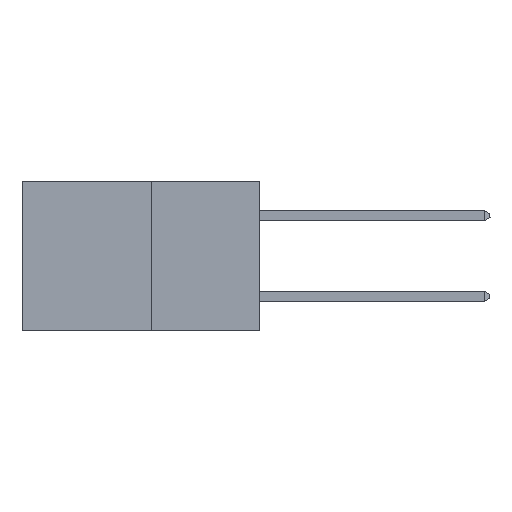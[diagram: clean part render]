
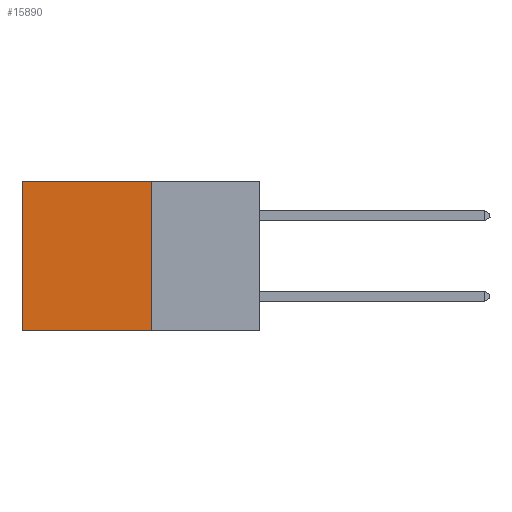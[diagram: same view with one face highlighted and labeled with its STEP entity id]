
A CAD part, left-side view. The second image highlights one B-rep face of the part: STEP entity #15890.
In plain terms, the highlighted planar face has unit normal (-1, 0, 0).
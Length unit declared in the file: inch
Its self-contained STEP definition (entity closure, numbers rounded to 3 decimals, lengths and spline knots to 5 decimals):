
#1110 = CARTESIAN_POINT ( 'NONE',  ( 0.277, 0.27, -0.37 ) ) ;
#1253 = AXIS2_PLACEMENT_3D ( 'NONE', #1110, #6618, #25514 ) ;
#2234 = CARTESIAN_POINT ( 'NONE',  ( 0.277, 0.59, 0. ) ) ;
#3628 = EDGE_CURVE ( 'NONE', #25313, #12297, #9365, .T. ) ;
#4826 = VECTOR ( 'NONE', #16252, 39.37008 ) ;
#4894 = DIRECTION ( 'NONE',  ( 0., 1., 0. ) ) ;
#5649 = LINE ( 'NONE', #13526, #4826 ) ;
#6618 = DIRECTION ( 'NONE',  ( 1., 0., 0. ) ) ;
#7846 = CARTESIAN_POINT ( 'NONE',  ( 0.277, 0.27, 0. ) ) ;
#9365 = LINE ( 'NONE', #32459, #22031 ) ;
#11184 = VECTOR ( 'NONE', #23980, 39.37008 ) ;
#11797 = LINE ( 'NONE', #29148, #25221 ) ;
#12297 = VERTEX_POINT ( 'NONE', #17534 ) ;
#13526 = CARTESIAN_POINT ( 'NONE',  ( 0.277, 0.27, -0.37 ) ) ;
#15696 = FACE_OUTER_BOUND ( 'NONE', #31262, .T. ) ;
#15890 = ADVANCED_FACE ( 'NONE', ( #15696 ), #22803, .F. ) ;
#16252 = DIRECTION ( 'NONE',  ( 0., 0., -1. ) ) ;
#17077 = ORIENTED_EDGE ( 'NONE', *, *, #31181, .F. ) ;
#17534 = CARTESIAN_POINT ( 'NONE',  ( 0.277, 0.59, -0.37 ) ) ;
#18004 = CARTESIAN_POINT ( 'NONE',  ( 0.277, 0.27, 0. ) ) ;
#19193 = LINE ( 'NONE', #7846, #11184 ) ;
#20995 = ORIENTED_EDGE ( 'NONE', *, *, #34697, .T. ) ;
#22031 = VECTOR ( 'NONE', #33277, 39.37008 ) ;
#22803 = PLANE ( 'NONE',  #1253 ) ;
#23266 = VERTEX_POINT ( 'NONE', #18004 ) ;
#23980 = DIRECTION ( 'NONE',  ( 0., 1., 0. ) ) ;
#25221 = VECTOR ( 'NONE', #4894, 39.37008 ) ;
#25313 = VERTEX_POINT ( 'NONE', #2234 ) ;
#25514 = DIRECTION ( 'NONE',  ( 0., 0., -1. ) ) ;
#28305 = ORIENTED_EDGE ( 'NONE', *, *, #3628, .T. ) ;
#29148 = CARTESIAN_POINT ( 'NONE',  ( 0.277, 0.27, -0.37 ) ) ;
#29630 = EDGE_CURVE ( 'NONE', #31920, #12297, #11797, .T. ) ;
#29732 = ORIENTED_EDGE ( 'NONE', *, *, #29630, .F. ) ;
#31181 = EDGE_CURVE ( 'NONE', #23266, #31920, #5649, .T. ) ;
#31262 = EDGE_LOOP ( 'NONE', ( #28305, #29732, #17077, #20995 ) ) ;
#31432 = CARTESIAN_POINT ( 'NONE',  ( 0.277, 0.27, -0.37 ) ) ;
#31920 = VERTEX_POINT ( 'NONE', #31432 ) ;
#32459 = CARTESIAN_POINT ( 'NONE',  ( 0.277, 0.59, -0.37 ) ) ;
#33277 = DIRECTION ( 'NONE',  ( 0., 0., -1. ) ) ;
#34697 = EDGE_CURVE ( 'NONE', #23266, #25313, #19193, .T. ) ;
